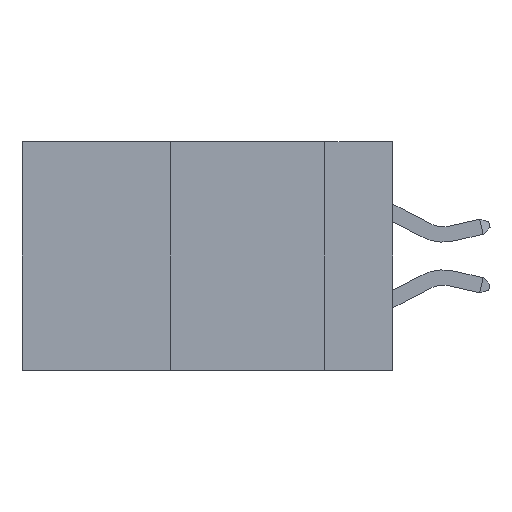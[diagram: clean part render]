
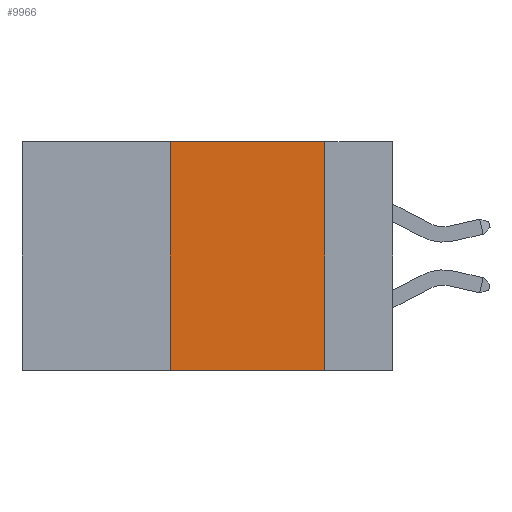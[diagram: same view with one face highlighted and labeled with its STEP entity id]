
A CAD part, left-side view. The second image highlights one B-rep face of the part: STEP entity #9966.
In plain terms, the highlighted planar face has unit normal (-1, 0, 0).
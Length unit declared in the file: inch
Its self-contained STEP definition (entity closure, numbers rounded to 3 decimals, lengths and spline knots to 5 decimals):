
#841 = VECTOR ( 'NONE', #9931, 39.37008 ) ;
#1192 = LINE ( 'NONE', #8169, #841 ) ;
#1318 = VERTEX_POINT ( 'NONE', #4639 ) ;
#1632 = VECTOR ( 'NONE', #9610, 39.37008 ) ;
#1683 = CARTESIAN_POINT ( 'NONE',  ( 0., 0.11, 0. ) ) ;
#1696 = DIRECTION ( 'NONE',  ( 1., 0., 0. ) ) ;
#1748 = LINE ( 'NONE', #6067, #1632 ) ;
#2176 = ORIENTED_EDGE ( 'NONE', *, *, #2869, .F. ) ;
#2557 = EDGE_CURVE ( 'NONE', #5783, #7412, #1192, .T. ) ;
#2869 = EDGE_CURVE ( 'NONE', #1318, #9255, #6022, .T. ) ;
#3302 = DIRECTION ( 'NONE',  ( 0., -1., 0. ) ) ;
#3489 = FACE_OUTER_BOUND ( 'NONE', #5087, .T. ) ;
#4580 = EDGE_CURVE ( 'NONE', #9255, #5783, #1748, .T. ) ;
#4639 = CARTESIAN_POINT ( 'NONE',  ( 0., 0.36, -0.37 ) ) ;
#5087 = EDGE_LOOP ( 'NONE', ( #7590, #8269, #2176, #5657 ) ) ;
#5657 = ORIENTED_EDGE ( 'NONE', *, *, #7576, .T. ) ;
#5783 = VERTEX_POINT ( 'NONE', #1683 ) ;
#5791 = CARTESIAN_POINT ( 'NONE',  ( 0., 0.11, -0.37 ) ) ;
#6022 = LINE ( 'NONE', #7129, #10435 ) ;
#6067 = CARTESIAN_POINT ( 'NONE',  ( 0., 0.6, 0. ) ) ;
#6864 = CARTESIAN_POINT ( 'NONE',  ( 0., 0.36, 0. ) ) ;
#6888 = CARTESIAN_POINT ( 'NONE',  ( 0., 0.6, 0. ) ) ;
#7129 = CARTESIAN_POINT ( 'NONE',  ( 0., 0.36, 0. ) ) ;
#7412 = VERTEX_POINT ( 'NONE', #5791 ) ;
#7576 = EDGE_CURVE ( 'NONE', #1318, #7412, #8788, .T. ) ;
#7590 = ORIENTED_EDGE ( 'NONE', *, *, #2557, .F. ) ;
#7790 = PLANE ( 'NONE',  #7958 ) ;
#7958 = AXIS2_PLACEMENT_3D ( 'NONE', #6888, #1696, #10495 ) ;
#8169 = CARTESIAN_POINT ( 'NONE',  ( 0., 0.11, 0. ) ) ;
#8269 = ORIENTED_EDGE ( 'NONE', *, *, #4580, .F. ) ;
#8788 = LINE ( 'NONE', #11362, #10644 ) ;
#9255 = VERTEX_POINT ( 'NONE', #6864 ) ;
#9610 = DIRECTION ( 'NONE',  ( 0., -1., 0. ) ) ;
#9931 = DIRECTION ( 'NONE',  ( 0., 0., -1. ) ) ;
#9966 = ADVANCED_FACE ( 'NONE', ( #3489 ), #7790, .F. ) ;
#10435 = VECTOR ( 'NONE', #10664, 39.37008 ) ;
#10495 = DIRECTION ( 'NONE',  ( 0., 0., -1. ) ) ;
#10644 = VECTOR ( 'NONE', #3302, 39.37008 ) ;
#10664 = DIRECTION ( 'NONE',  ( 0., 0., 1. ) ) ;
#11362 = CARTESIAN_POINT ( 'NONE',  ( 0., 0.6, -0.37 ) ) ;
